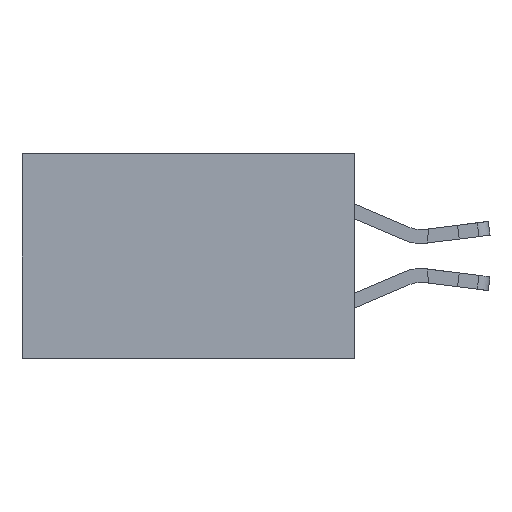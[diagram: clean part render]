
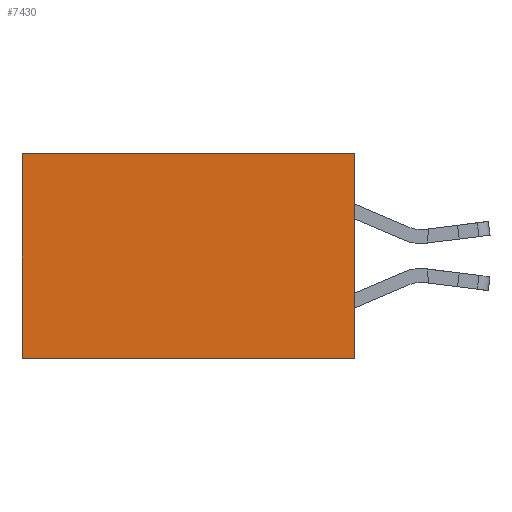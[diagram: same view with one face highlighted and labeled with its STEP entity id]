
A CAD part, left-side view. The second image highlights one B-rep face of the part: STEP entity #7430.
In plain terms, the highlighted planar face has unit normal (-1, 0, 0).
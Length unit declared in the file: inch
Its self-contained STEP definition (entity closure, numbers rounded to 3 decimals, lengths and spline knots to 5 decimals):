
#436 = CARTESIAN_POINT ( 'NONE',  ( 0.2615, 0., 0. ) ) ;
#1469 = ORIENTED_EDGE ( 'NONE', *, *, #10107, .T. ) ;
#1499 = LINE ( 'NONE', #436, #6846 ) ;
#1527 = VECTOR ( 'NONE', #12371, 39.37008 ) ;
#1664 = ORIENTED_EDGE ( 'NONE', *, *, #8452, .F. ) ;
#2211 = VERTEX_POINT ( 'NONE', #11376 ) ;
#2256 = VECTOR ( 'NONE', #5214, 39.37008 ) ;
#2355 = AXIS2_PLACEMENT_3D ( 'NONE', #8257, #11425, #10495 ) ;
#2887 = CARTESIAN_POINT ( 'NONE',  ( 0.2615, 0., -0.37 ) ) ;
#3437 = CARTESIAN_POINT ( 'NONE',  ( 0.2615, 0., -0.37 ) ) ;
#4539 = DIRECTION ( 'NONE',  ( 0., 0., -1. ) ) ;
#5172 = EDGE_CURVE ( 'NONE', #5875, #2211, #9097, .T. ) ;
#5214 = DIRECTION ( 'NONE',  ( 0., 1., 0. ) ) ;
#5744 = CARTESIAN_POINT ( 'NONE',  ( 0.2615, 0.6, -0.37 ) ) ;
#5875 = VERTEX_POINT ( 'NONE', #12943 ) ;
#6648 = VERTEX_POINT ( 'NONE', #12607 ) ;
#6846 = VECTOR ( 'NONE', #13645, 39.37008 ) ;
#7249 = LINE ( 'NONE', #2887, #2256 ) ;
#7430 = ADVANCED_FACE ( 'NONE', ( #13655 ), #10279, .F. ) ;
#8257 = CARTESIAN_POINT ( 'NONE',  ( 0.2615, 0., -0.37 ) ) ;
#8452 = EDGE_CURVE ( 'NONE', #2211, #6648, #7249, .T. ) ;
#8725 = LINE ( 'NONE', #5744, #1527 ) ;
#8845 = CARTESIAN_POINT ( 'NONE',  ( 0.2615, 0.6, 0. ) ) ;
#9097 = LINE ( 'NONE', #3437, #12765 ) ;
#10107 = EDGE_CURVE ( 'NONE', #5875, #12341, #1499, .T. ) ;
#10279 = PLANE ( 'NONE',  #2355 ) ;
#10495 = DIRECTION ( 'NONE',  ( 0., 0., -1. ) ) ;
#10722 = EDGE_CURVE ( 'NONE', #12341, #6648, #8725, .T. ) ;
#11152 = EDGE_LOOP ( 'NONE', ( #14206, #1664, #11784, #1469 ) ) ;
#11376 = CARTESIAN_POINT ( 'NONE',  ( 0.2615, 0., -0.37 ) ) ;
#11425 = DIRECTION ( 'NONE',  ( 1., 0., 0. ) ) ;
#11784 = ORIENTED_EDGE ( 'NONE', *, *, #5172, .F. ) ;
#12341 = VERTEX_POINT ( 'NONE', #8845 ) ;
#12371 = DIRECTION ( 'NONE',  ( 0., 0., -1. ) ) ;
#12607 = CARTESIAN_POINT ( 'NONE',  ( 0.2615, 0.6, -0.37 ) ) ;
#12765 = VECTOR ( 'NONE', #4539, 39.37008 ) ;
#12943 = CARTESIAN_POINT ( 'NONE',  ( 0.2615, 0., 0. ) ) ;
#13645 = DIRECTION ( 'NONE',  ( 0., 1., 0. ) ) ;
#13655 = FACE_OUTER_BOUND ( 'NONE', #11152, .T. ) ;
#14206 = ORIENTED_EDGE ( 'NONE', *, *, #10722, .T. ) ;
